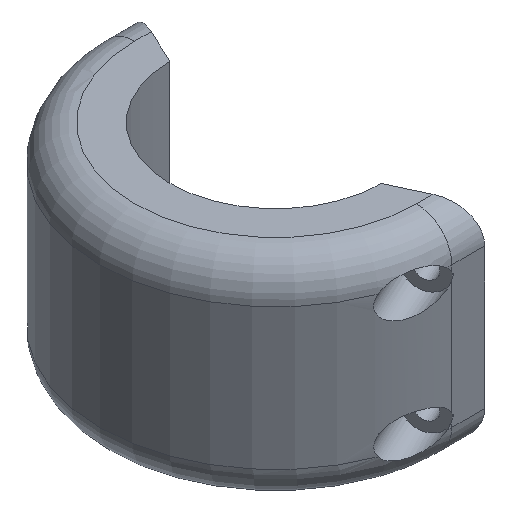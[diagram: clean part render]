
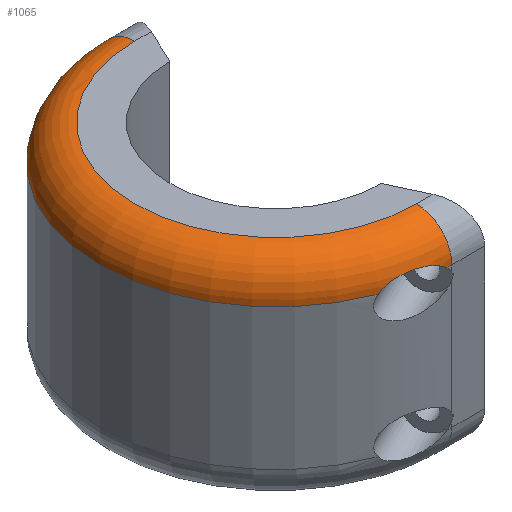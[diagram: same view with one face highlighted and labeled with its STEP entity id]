
A CAD part, isometric view. The second image highlights one B-rep face of the part: STEP entity #1065.
In plain terms, the highlighted toroidal (fillet/blend) face has major radius 25.4 mm and minor radius 6.35 mm.
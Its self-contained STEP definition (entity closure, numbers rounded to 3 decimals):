
#26 = CARTESIAN_POINT ( 'NONE',  ( -50.8, -25.4, 12.7 ) ) ;
#29 = CARTESIAN_POINT ( 'NONE',  ( -53.279, -31.572, 7.369 ) ) ;
#33 = CARTESIAN_POINT ( 'NONE',  ( -60.143, -30.199, 7.692 ) ) ;
#37 = EDGE_CURVE ( 'NONE', #806, #259, #824, .T. ) ;
#38 = CARTESIAN_POINT ( 'NONE',  ( -53.714, 31.501, 7.56 ) ) ;
#41 = CARTESIAN_POINT ( 'NONE',  ( -60.577, 30.102, 7.513 ) ) ;
#49 = CARTESIAN_POINT ( 'NONE',  ( -62.04, 29.694, 6.35 ) ) ;
#80 = AXIS2_PLACEMENT_3D ( 'NONE', #395, #335, #331 ) ;
#100 = EDGE_CURVE ( 'NONE', #228, #443, #785, .T. ) ;
#102 = CARTESIAN_POINT ( 'NONE',  ( -50.8, 25.4, 12.7 ) ) ;
#118 = CARTESIAN_POINT ( 'NONE',  ( -50.8, 0., 6.35 ) ) ;
#119 = DIRECTION ( 'NONE',  ( 1., 0., 0. ) ) ;
#120 = CARTESIAN_POINT ( 'NONE',  ( -53.937, -31.462, 7.646 ) ) ;
#123 = CARTESIAN_POINT ( 'NONE',  ( -61.188, -29.95, 7.153 ) ) ;
#125 = VERTEX_POINT ( 'NONE', #1054 ) ;
#129 = CARTESIAN_POINT ( 'NONE',  ( -54.606, 31.339, 7.874 ) ) ;
#132 = CARTESIAN_POINT ( 'NONE',  ( -61.381, 29.9, 7.019 ) ) ;
#134 = DIRECTION ( 'NONE',  ( 1., 0., 0. ) ) ;
#137 = DIRECTION ( 'NONE',  ( 0., 0., -1. ) ) ;
#143 = CARTESIAN_POINT ( 'NONE',  ( -50.8, 0., 6.35 ) ) ;
#175 = CARTESIAN_POINT ( 'NONE',  ( -50.8, 0., 12.7 ) ) ;
#187 = CARTESIAN_POINT ( 'NONE',  ( -51.675, -31.738, 6.35 ) ) ;
#191 = DIRECTION ( 'NONE',  ( 1., 0., 0. ) ) ;
#194 = CARTESIAN_POINT ( 'NONE',  ( -55.06, -31.25, 7.987 ) ) ;
#196 = CARTESIAN_POINT ( 'NONE',  ( -61.737, -29.798, 6.715 ) ) ;
#198 = CARTESIAN_POINT ( 'NONE',  ( -51.675, 31.738, 6.35 ) ) ;
#201 = CARTESIAN_POINT ( 'NONE',  ( -55.75, 31.112, 8.105 ) ) ;
#205 = CARTESIAN_POINT ( 'NONE',  ( -61.902, 29.746, 6.543 ) ) ;
#224 = AXIS2_PLACEMENT_3D ( 'NONE', #1015, #596, #119 ) ;
#228 = VERTEX_POINT ( 'NONE', #999 ) ;
#259 = VERTEX_POINT ( 'NONE', #488 ) ;
#260 = AXIS2_PLACEMENT_3D ( 'NONE', #901, #332, #1007 ) ;
#262 = CARTESIAN_POINT ( 'NONE',  ( -51.675, -31.738, 6.35 ) ) ;
#264 = CARTESIAN_POINT ( 'NONE',  ( -55.982, -31.065, 8.136 ) ) ;
#267 = CARTESIAN_POINT ( 'NONE',  ( -62.04, -29.694, 6.35 ) ) ;
#274 = CARTESIAN_POINT ( 'NONE',  ( -56.45, 30.97, 8.18 ) ) ;
#307 = AXIS2_PLACEMENT_3D ( 'NONE', #118, #698, #191 ) ;
#312 = EDGE_CURVE ( 'NONE', #1009, #259, #703, .T. ) ;
#331 = DIRECTION ( 'NONE',  ( 1., 0., 0. ) ) ;
#332 = DIRECTION ( 'NONE',  ( 1., 0., 0. ) ) ;
#335 = DIRECTION ( 'NONE',  ( 0., 0., -1. ) ) ;
#340 = CARTESIAN_POINT ( 'NONE',  ( -52.049, -31.728, 6.657 ) ) ;
#344 = CARTESIAN_POINT ( 'NONE',  ( -56.686, -30.922, 8.193 ) ) ;
#353 = AXIS2_PLACEMENT_3D ( 'NONE', #143, #137, #134 ) ;
#354 = CARTESIAN_POINT ( 'NONE',  ( -57.39, 30.778, 8.207 ) ) ;
#371 = EDGE_CURVE ( 'NONE', #1009, #496, #720, .T. ) ;
#395 = CARTESIAN_POINT ( 'NONE',  ( -50.8, 0., 6.35 ) ) ;
#420 = CARTESIAN_POINT ( 'NONE',  ( -57.856, -30.683, 8.183 ) ) ;
#422 = EDGE_CURVE ( 'NONE', #496, #125, #688, .T. ) ;
#429 = CARTESIAN_POINT ( 'NONE',  ( -52.444, 31.689, 6.922 ) ) ;
#434 = CARTESIAN_POINT ( 'NONE',  ( -58.781, 30.491, 8.064 ) ) ;
#443 = VERTEX_POINT ( 'NONE', #49 ) ;
#451 = ORIENTED_EDGE ( 'NONE', *, *, #422, .F. ) ;
#453 = ORIENTED_EDGE ( 'NONE', *, *, #371, .F. ) ;
#460 = B_SPLINE_CURVE_WITH_KNOTS ( 'NONE', 3,
 ( #198, #710, #429, #1132, #519, #38, #609, #129, #716, #201, #815, #274, #931, #354, #1033, #434, #1137, #522, #41, #616, #132, #719, #205, #821 ),
 .UNSPECIFIED., .F., .F.,
 ( 4, 2, 2, 2, 2, 2, 2, 2, 2, 2, 2, 4 ),
 ( 0., 0.001, 0.002, 0.003, 0.004, 0.005, 0.006, 0.007, 0.009, 0.01, 0.011, 0.011 ),
 .UNSPECIFIED. ) ;
#463 = DIRECTION ( 'NONE',  ( 1., 0., 0. ) ) ;
#469 = VERTEX_POINT ( 'NONE', #187 ) ;
#475 = EDGE_CURVE ( 'NONE', #125, #469, #670, .T. ) ;
#482 = DIRECTION ( 'NONE',  ( 0., 0., 1. ) ) ;
#488 = CARTESIAN_POINT ( 'NONE',  ( -50.8, 31.75, 6.35 ) ) ;
#495 = FACE_OUTER_BOUND ( 'NONE', #894, .T. ) ;
#496 = VERTEX_POINT ( 'NONE', #26 ) ;
#501 = TOROIDAL_SURFACE ( 'NONE', #224, 25.4, 6.35 ) ;
#504 = B_SPLINE_CURVE_WITH_KNOTS ( 'NONE', 3,
 ( #262, #340, #1120, #508, #29, #600, #120, #700, #194, #805, #264, #918, #344, #1018, #420, #1127, #511, #33, #604, #123, #704, #196, #810, #267 ),
 .UNSPECIFIED., .F., .F.,
 ( 4, 2, 2, 2, 2, 2, 2, 2, 2, 2, 2, 4 ),
 ( 0., 0.001, 0.002, 0.003, 0.004, 0.005, 0.006, 0.007, 0.009, 0.01, 0.011, 0.011 ),
 .UNSPECIFIED. ) ;
#508 = CARTESIAN_POINT ( 'NONE',  ( -53.067, -31.604, 7.264 ) ) ;
#511 = CARTESIAN_POINT ( 'NONE',  ( -59.241, -30.395, 7.969 ) ) ;
#519 = CARTESIAN_POINT ( 'NONE',  ( -53.279, 31.572, 7.369 ) ) ;
#522 = CARTESIAN_POINT ( 'NONE',  ( -60.143, 30.199, 7.692 ) ) ;
#543 = EDGE_CURVE ( 'NONE', #469, #228, #504, .T. ) ;
#596 = DIRECTION ( 'NONE',  ( 0., 0., 1. ) ) ;
#600 = CARTESIAN_POINT ( 'NONE',  ( -53.714, -31.501, 7.56 ) ) ;
#601 = DIRECTION ( 'NONE',  ( 0., 0., 1. ) ) ;
#604 = CARTESIAN_POINT ( 'NONE',  ( -60.577, -30.102, 7.513 ) ) ;
#606 = EDGE_CURVE ( 'NONE', #806, #443, #460, .T. ) ;
#609 = CARTESIAN_POINT ( 'NONE',  ( -53.937, 31.462, 7.646 ) ) ;
#616 = CARTESIAN_POINT ( 'NONE',  ( -61.188, 29.95, 7.153 ) ) ;
#670 = CIRCLE ( 'NONE', #307, 31.75 ) ;
#688 = CIRCLE ( 'NONE', #260, 6.35 ) ;
#693 = DIRECTION ( 'NONE',  ( -1., 0., 0. ) ) ;
#698 = DIRECTION ( 'NONE',  ( 0., 0., -1. ) ) ;
#700 = CARTESIAN_POINT ( 'NONE',  ( -54.606, -31.339, 7.874 ) ) ;
#701 = CARTESIAN_POINT ( 'NONE',  ( -50.8, 25.4, 6.35 ) ) ;
#703 = CIRCLE ( 'NONE', #1116, 6.35 ) ;
#704 = CARTESIAN_POINT ( 'NONE',  ( -61.381, -29.9, 7.019 ) ) ;
#710 = CARTESIAN_POINT ( 'NONE',  ( -52.049, 31.728, 6.657 ) ) ;
#716 = CARTESIAN_POINT ( 'NONE',  ( -55.06, 31.25, 7.987 ) ) ;
#719 = CARTESIAN_POINT ( 'NONE',  ( -61.737, 29.798, 6.715 ) ) ;
#720 = CIRCLE ( 'NONE', #1046, 25.4 ) ;
#785 = CIRCLE ( 'NONE', #80, 31.75 ) ;
#805 = CARTESIAN_POINT ( 'NONE',  ( -55.75, -31.112, 8.105 ) ) ;
#806 = VERTEX_POINT ( 'NONE', #949 ) ;
#810 = CARTESIAN_POINT ( 'NONE',  ( -61.902, -29.746, 6.543 ) ) ;
#815 = CARTESIAN_POINT ( 'NONE',  ( -55.982, 31.065, 8.136 ) ) ;
#821 = CARTESIAN_POINT ( 'NONE',  ( -62.04, 29.694, 6.35 ) ) ;
#824 = CIRCLE ( 'NONE', #353, 31.75 ) ;
#894 = EDGE_LOOP ( 'NONE', ( #1135, #1139, #1148, #1149, #1155, #451, #453, #1158 ) ) ;
#901 = CARTESIAN_POINT ( 'NONE',  ( -50.8, -25.4, 6.35 ) ) ;
#918 = CARTESIAN_POINT ( 'NONE',  ( -56.45, -30.97, 8.18 ) ) ;
#931 = CARTESIAN_POINT ( 'NONE',  ( -56.686, 30.922, 8.193 ) ) ;
#949 = CARTESIAN_POINT ( 'NONE',  ( -51.675, 31.738, 6.35 ) ) ;
#999 = CARTESIAN_POINT ( 'NONE',  ( -62.04, -29.694, 6.35 ) ) ;
#1007 = DIRECTION ( 'NONE',  ( 0., 0., -1. ) ) ;
#1009 = VERTEX_POINT ( 'NONE', #102 ) ;
#1015 = CARTESIAN_POINT ( 'NONE',  ( -50.8, 0., 6.35 ) ) ;
#1018 = CARTESIAN_POINT ( 'NONE',  ( -57.39, -30.778, 8.207 ) ) ;
#1033 = CARTESIAN_POINT ( 'NONE',  ( -57.856, 30.683, 8.183 ) ) ;
#1046 = AXIS2_PLACEMENT_3D ( 'NONE', #175, #482, #463 ) ;
#1054 = CARTESIAN_POINT ( 'NONE',  ( -50.8, -31.75, 6.35 ) ) ;
#1065 = ADVANCED_FACE ( 'NONE', ( #495 ), #501, .T. ) ;
#1116 = AXIS2_PLACEMENT_3D ( 'NONE', #701, #693, #601 ) ;
#1120 = CARTESIAN_POINT ( 'NONE',  ( -52.444, -31.689, 6.922 ) ) ;
#1127 = CARTESIAN_POINT ( 'NONE',  ( -58.781, -30.491, 8.064 ) ) ;
#1132 = CARTESIAN_POINT ( 'NONE',  ( -53.067, 31.604, 7.264 ) ) ;
#1135 = ORIENTED_EDGE ( 'NONE', *, *, #37, .F. ) ;
#1137 = CARTESIAN_POINT ( 'NONE',  ( -59.241, 30.395, 7.969 ) ) ;
#1139 = ORIENTED_EDGE ( 'NONE', *, *, #606, .T. ) ;
#1148 = ORIENTED_EDGE ( 'NONE', *, *, #100, .F. ) ;
#1149 = ORIENTED_EDGE ( 'NONE', *, *, #543, .F. ) ;
#1155 = ORIENTED_EDGE ( 'NONE', *, *, #475, .F. ) ;
#1158 = ORIENTED_EDGE ( 'NONE', *, *, #312, .T. ) ;
